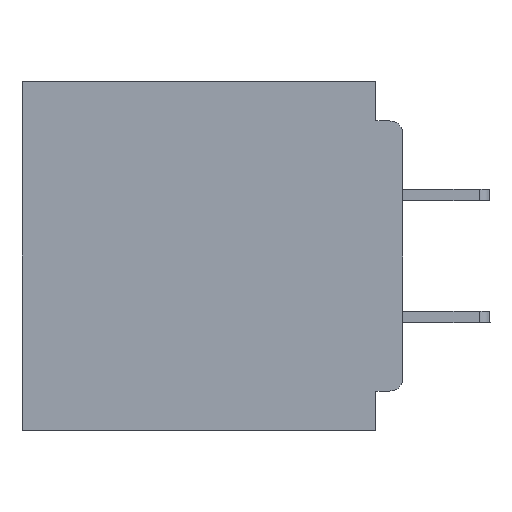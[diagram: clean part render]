
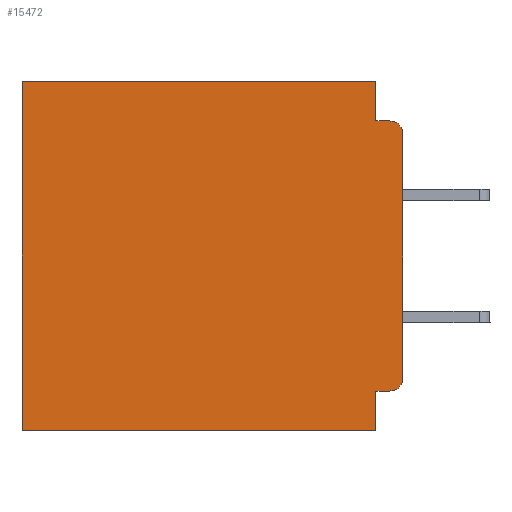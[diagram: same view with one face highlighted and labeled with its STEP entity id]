
A CAD part, left-side view. The second image highlights one B-rep face of the part: STEP entity #15472.
In plain terms, the highlighted planar face has unit normal (-1, 0, 0).
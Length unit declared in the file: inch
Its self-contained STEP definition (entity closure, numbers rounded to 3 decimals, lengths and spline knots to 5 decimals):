
#204 = DIRECTION ( 'NONE',  ( 0., 0., -1. ) ) ;
#553 = DIRECTION ( 'NONE',  ( 0., 0., -1. ) ) ;
#1198 = VERTEX_POINT ( 'NONE', #45764 ) ;
#4741 = EDGE_LOOP ( 'NONE', ( #31046, #24596, #47435, #42610, #18448, #5532, #40545, #58276, #7662, #47056 ) ) ;
#5100 = LINE ( 'NONE', #11817, #28089 ) ;
#5167 = VERTEX_POINT ( 'NONE', #17493 ) ;
#5532 = ORIENTED_EDGE ( 'NONE', *, *, #54776, .T. ) ;
#5562 = EDGE_CURVE ( 'NONE', #49098, #31563, #35505, .T. ) ;
#5640 = LINE ( 'NONE', #15169, #27200 ) ;
#6701 = EDGE_CURVE ( 'NONE', #30200, #1198, #58162, .T. ) ;
#7662 = ORIENTED_EDGE ( 'NONE', *, *, #6701, .F. ) ;
#8321 = CARTESIAN_POINT ( 'NONE',  ( 0.3, 0.031, 0. ) ) ;
#8461 = CARTESIAN_POINT ( 'NONE',  ( 0.3, 0.015, -0.06 ) ) ;
#9487 = DIRECTION ( 'NONE',  ( 0., -1., 0. ) ) ;
#10118 = VECTOR ( 'NONE', #35845, 39.37008 ) ;
#11566 = LINE ( 'NONE', #8321, #10118 ) ;
#11817 = CARTESIAN_POINT ( 'NONE',  ( 0.3, 0.031, -0.4 ) ) ;
#13085 = DIRECTION ( 'NONE',  ( 0., 0., -1. ) ) ;
#13908 = CARTESIAN_POINT ( 'NONE',  ( 0.3, 0.031, 0. ) ) ;
#14484 = CARTESIAN_POINT ( 'NONE',  ( 0.3, 0.031, -0.045 ) ) ;
#15132 = LINE ( 'NONE', #32387, #36695 ) ;
#15169 = CARTESIAN_POINT ( 'NONE',  ( 0.3, 0.437, -0.4 ) ) ;
#15394 = CIRCLE ( 'NONE', #53226, 0.015 ) ;
#15472 = ADVANCED_FACE ( 'NONE', ( #18359 ), #54921, .F. ) ;
#15534 = DIRECTION ( 'NONE',  ( 0., 1., 0. ) ) ;
#17493 = CARTESIAN_POINT ( 'NONE',  ( 0.3, 0.437, 0. ) ) ;
#18025 = VECTOR ( 'NONE', #45522, 39.37008 ) ;
#18359 = FACE_OUTER_BOUND ( 'NONE', #4741, .T. ) ;
#18448 = ORIENTED_EDGE ( 'NONE', *, *, #34348, .T. ) ;
#19805 = DIRECTION ( 'NONE',  ( 0., 0., -1. ) ) ;
#20785 = EDGE_CURVE ( 'NONE', #36754, #52156, #52308, .T. ) ;
#24596 = ORIENTED_EDGE ( 'NONE', *, *, #53798, .T. ) ;
#26339 = EDGE_CURVE ( 'NONE', #30200, #31563, #15394, .T. ) ;
#27200 = VECTOR ( 'NONE', #19805, 39.37008 ) ;
#27665 = DIRECTION ( 'NONE',  ( 1., 0., 0. ) ) ;
#28004 = DIRECTION ( 'NONE',  ( -1., 0., 0. ) ) ;
#28089 = VECTOR ( 'NONE', #48423, 39.37008 ) ;
#29043 = CARTESIAN_POINT ( 'NONE',  ( 0.3, 0., -0.34 ) ) ;
#29218 = CARTESIAN_POINT ( 'NONE',  ( 0.3, 0., -0.355 ) ) ;
#30200 = VERTEX_POINT ( 'NONE', #36218 ) ;
#30264 = LINE ( 'NONE', #31794, #18025 ) ;
#30362 = VERTEX_POINT ( 'NONE', #14484 ) ;
#31046 = ORIENTED_EDGE ( 'NONE', *, *, #5562, .F. ) ;
#31563 = VERTEX_POINT ( 'NONE', #29043 ) ;
#31794 = CARTESIAN_POINT ( 'NONE',  ( 0.3, 0., 0. ) ) ;
#32387 = CARTESIAN_POINT ( 'NONE',  ( 0.3, 0., -0.045 ) ) ;
#33465 = EDGE_CURVE ( 'NONE', #1198, #36754, #5100, .T. ) ;
#34271 = EDGE_CURVE ( 'NONE', #37397, #30362, #11566, .T. ) ;
#34348 = EDGE_CURVE ( 'NONE', #37397, #5167, #30264, .T. ) ;
#34438 = EDGE_CURVE ( 'NONE', #30362, #45031, #15132, .T. ) ;
#34528 = CIRCLE ( 'NONE', #41434, 0.015 ) ;
#35505 = LINE ( 'NONE', #40576, #44709 ) ;
#35845 = DIRECTION ( 'NONE',  ( 0., 0., -1. ) ) ;
#36218 = CARTESIAN_POINT ( 'NONE',  ( 0.3, 0.015, -0.355 ) ) ;
#36695 = VECTOR ( 'NONE', #9487, 39.37008 ) ;
#36754 = VERTEX_POINT ( 'NONE', #49974 ) ;
#36761 = CARTESIAN_POINT ( 'NONE',  ( 0.3, 0.437, -0.4 ) ) ;
#37397 = VERTEX_POINT ( 'NONE', #13908 ) ;
#40277 = VECTOR ( 'NONE', #53904, 39.37008 ) ;
#40545 = ORIENTED_EDGE ( 'NONE', *, *, #20785, .F. ) ;
#40570 = DIRECTION ( 'NONE',  ( -1., 0., 0. ) ) ;
#40576 = CARTESIAN_POINT ( 'NONE',  ( 0.3, 0., -0.4 ) ) ;
#41434 = AXIS2_PLACEMENT_3D ( 'NONE', #8461, #40570, #13085 ) ;
#42610 = ORIENTED_EDGE ( 'NONE', *, *, #34271, .F. ) ;
#42960 = CARTESIAN_POINT ( 'NONE',  ( 0.3, 0.015, -0.045 ) ) ;
#44709 = VECTOR ( 'NONE', #56766, 39.37008 ) ;
#45031 = VERTEX_POINT ( 'NONE', #42960 ) ;
#45522 = DIRECTION ( 'NONE',  ( 0., 1., 0. ) ) ;
#45764 = CARTESIAN_POINT ( 'NONE',  ( 0.3, 0.031, -0.355 ) ) ;
#45792 = CARTESIAN_POINT ( 'NONE',  ( 0.3, 0., -0.4 ) ) ;
#47056 = ORIENTED_EDGE ( 'NONE', *, *, #26339, .T. ) ;
#47435 = ORIENTED_EDGE ( 'NONE', *, *, #34438, .F. ) ;
#48423 = DIRECTION ( 'NONE',  ( 0., 0., -1. ) ) ;
#49098 = VERTEX_POINT ( 'NONE', #49491 ) ;
#49364 = CARTESIAN_POINT ( 'NONE',  ( 0.3, 0., -0.4 ) ) ;
#49491 = CARTESIAN_POINT ( 'NONE',  ( 0.3, 0., -0.06 ) ) ;
#49974 = CARTESIAN_POINT ( 'NONE',  ( 0.3, 0.031, -0.4 ) ) ;
#52156 = VERTEX_POINT ( 'NONE', #36761 ) ;
#52308 = LINE ( 'NONE', #49364, #40277 ) ;
#53226 = AXIS2_PLACEMENT_3D ( 'NONE', #55265, #28004, #553 ) ;
#53798 = EDGE_CURVE ( 'NONE', #49098, #45031, #34528, .T. ) ;
#53904 = DIRECTION ( 'NONE',  ( 0., 1., 0. ) ) ;
#54776 = EDGE_CURVE ( 'NONE', #5167, #52156, #5640, .T. ) ;
#54921 = PLANE ( 'NONE',  #57408 ) ;
#55265 = CARTESIAN_POINT ( 'NONE',  ( 0.3, 0.015, -0.34 ) ) ;
#56734 = VECTOR ( 'NONE', #15534, 39.37008 ) ;
#56766 = DIRECTION ( 'NONE',  ( 0., 0., -1. ) ) ;
#57408 = AXIS2_PLACEMENT_3D ( 'NONE', #45792, #27665, #204 ) ;
#58162 = LINE ( 'NONE', #29218, #56734 ) ;
#58276 = ORIENTED_EDGE ( 'NONE', *, *, #33465, .F. ) ;
